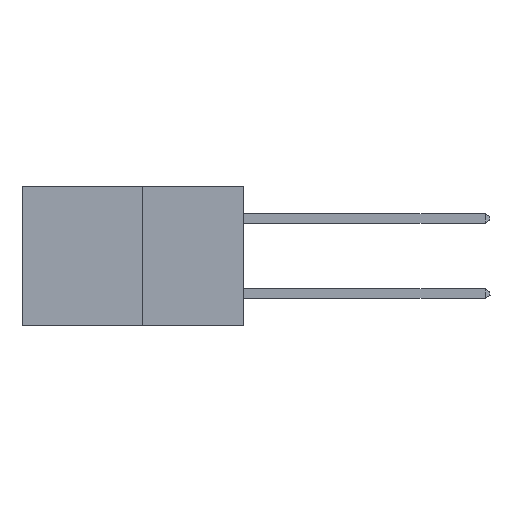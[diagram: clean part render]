
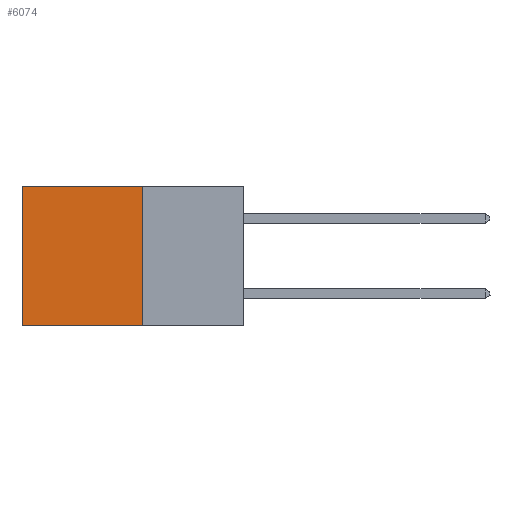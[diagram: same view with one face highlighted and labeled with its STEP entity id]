
A CAD part, left-side view. The second image highlights one B-rep face of the part: STEP entity #6074.
In plain terms, the highlighted planar face has unit normal (-1, 0, 0).
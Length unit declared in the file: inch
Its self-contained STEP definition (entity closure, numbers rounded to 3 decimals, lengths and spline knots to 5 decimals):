
#88 = AXIS2_PLACEMENT_3D ( 'NONE', #7751, #8469, #4318 ) ;
#300 = VERTEX_POINT ( 'NONE', #8108 ) ;
#542 = ORIENTED_EDGE ( 'NONE', *, *, #4609, .T. ) ;
#901 = VECTOR ( 'NONE', #5508, 39.37008 ) ;
#944 = ORIENTED_EDGE ( 'NONE', *, *, #1545, .F. ) ;
#955 = EDGE_CURVE ( 'NONE', #7970, #300, #7172, .T. ) ;
#1147 = EDGE_CURVE ( 'NONE', #3174, #300, #3679, .T. ) ;
#1200 = VECTOR ( 'NONE', #4962, 39.37008 ) ;
#1545 = EDGE_CURVE ( 'NONE', #6231, #3174, #5988, .T. ) ;
#1801 = DIRECTION ( 'NONE',  ( 0., 1., 0. ) ) ;
#3174 = VERTEX_POINT ( 'NONE', #9401 ) ;
#3198 = LINE ( 'NONE', #5540, #901 ) ;
#3527 = CARTESIAN_POINT ( 'NONE',  ( 0.277, 0.27, -0.37 ) ) ;
#3679 = LINE ( 'NONE', #3527, #8929 ) ;
#4318 = DIRECTION ( 'NONE',  ( 0., 0., -1. ) ) ;
#4609 = EDGE_CURVE ( 'NONE', #6231, #7970, #3198, .T. ) ;
#4687 = FACE_OUTER_BOUND ( 'NONE', #5063, .T. ) ;
#4818 = CARTESIAN_POINT ( 'NONE',  ( 0.277, 0.59, 0. ) ) ;
#4962 = DIRECTION ( 'NONE',  ( 0., 0., -1. ) ) ;
#5063 = EDGE_LOOP ( 'NONE', ( #7795, #8883, #944, #542 ) ) ;
#5508 = DIRECTION ( 'NONE',  ( 0., 1., 0. ) ) ;
#5540 = CARTESIAN_POINT ( 'NONE',  ( 0.277, 0.27, 0. ) ) ;
#5988 = LINE ( 'NONE', #7255, #7363 ) ;
#6074 = ADVANCED_FACE ( 'NONE', ( #4687 ), #7784, .F. ) ;
#6231 = VERTEX_POINT ( 'NONE', #8681 ) ;
#6516 = CARTESIAN_POINT ( 'NONE',  ( 0.277, 0.59, -0.37 ) ) ;
#7172 = LINE ( 'NONE', #6516, #1200 ) ;
#7255 = CARTESIAN_POINT ( 'NONE',  ( 0.277, 0.27, -0.37 ) ) ;
#7363 = VECTOR ( 'NONE', #8265, 39.37008 ) ;
#7751 = CARTESIAN_POINT ( 'NONE',  ( 0.277, 0.27, -0.37 ) ) ;
#7784 = PLANE ( 'NONE',  #88 ) ;
#7795 = ORIENTED_EDGE ( 'NONE', *, *, #955, .T. ) ;
#7970 = VERTEX_POINT ( 'NONE', #4818 ) ;
#8108 = CARTESIAN_POINT ( 'NONE',  ( 0.277, 0.59, -0.37 ) ) ;
#8265 = DIRECTION ( 'NONE',  ( 0., 0., -1. ) ) ;
#8469 = DIRECTION ( 'NONE',  ( 1., 0., 0. ) ) ;
#8681 = CARTESIAN_POINT ( 'NONE',  ( 0.277, 0.27, 0. ) ) ;
#8883 = ORIENTED_EDGE ( 'NONE', *, *, #1147, .F. ) ;
#8929 = VECTOR ( 'NONE', #1801, 39.37008 ) ;
#9401 = CARTESIAN_POINT ( 'NONE',  ( 0.277, 0.27, -0.37 ) ) ;
